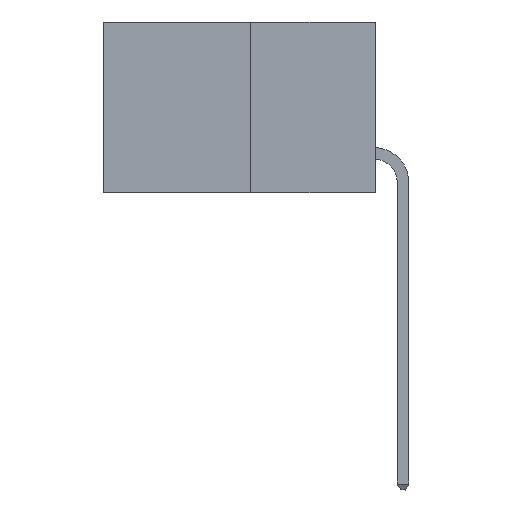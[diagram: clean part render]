
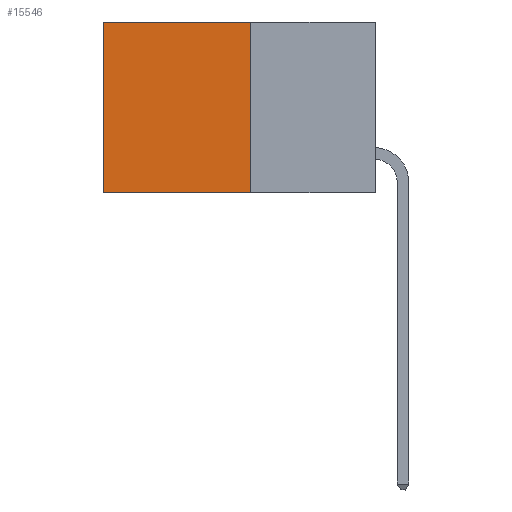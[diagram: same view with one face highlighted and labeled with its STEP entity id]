
A CAD part, left-side view. The second image highlights one B-rep face of the part: STEP entity #15546.
In plain terms, the highlighted planar face has unit normal (-1, 0, 0).
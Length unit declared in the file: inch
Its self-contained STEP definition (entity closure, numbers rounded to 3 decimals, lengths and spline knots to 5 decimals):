
#466 = DIRECTION ( 'NONE',  ( 0., 0., -1. ) ) ;
#811 = CARTESIAN_POINT ( 'NONE',  ( 0.277, 0.27, -0.37 ) ) ;
#1343 = VERTEX_POINT ( 'NONE', #15379 ) ;
#1377 = CARTESIAN_POINT ( 'NONE',  ( 0.277, 0.27, 0. ) ) ;
#2199 = DIRECTION ( 'NONE',  ( 0., 0., -1. ) ) ;
#2752 = EDGE_CURVE ( 'NONE', #14005, #12469, #15935, .T. ) ;
#4328 = VECTOR ( 'NONE', #6142, 39.37008 ) ;
#4479 = LINE ( 'NONE', #12150, #11175 ) ;
#4634 = EDGE_CURVE ( 'NONE', #8084, #1343, #10798, .T. ) ;
#4691 = CARTESIAN_POINT ( 'NONE',  ( 0.277, 0.27, -0.37 ) ) ;
#4989 = AXIS2_PLACEMENT_3D ( 'NONE', #811, #9878, #2199 ) ;
#5261 = ORIENTED_EDGE ( 'NONE', *, *, #2752, .F. ) ;
#5404 = EDGE_CURVE ( 'NONE', #8084, #14005, #16242, .T. ) ;
#5988 = ORIENTED_EDGE ( 'NONE', *, *, #4634, .T. ) ;
#6006 = ORIENTED_EDGE ( 'NONE', *, *, #5404, .F. ) ;
#6142 = DIRECTION ( 'NONE',  ( 0., 1., 0. ) ) ;
#7275 = ORIENTED_EDGE ( 'NONE', *, *, #8426, .T. ) ;
#8084 = VERTEX_POINT ( 'NONE', #1377 ) ;
#8426 = EDGE_CURVE ( 'NONE', #1343, #12469, #4479, .T. ) ;
#9634 = DIRECTION ( 'NONE',  ( 0., 0., -1. ) ) ;
#9728 = CARTESIAN_POINT ( 'NONE',  ( 0.277, 0.59, -0.37 ) ) ;
#9786 = VECTOR ( 'NONE', #9634, 39.37008 ) ;
#9875 = FACE_OUTER_BOUND ( 'NONE', #14881, .T. ) ;
#9878 = DIRECTION ( 'NONE',  ( 1., 0., 0. ) ) ;
#10403 = VECTOR ( 'NONE', #14454, 39.37008 ) ;
#10744 = CARTESIAN_POINT ( 'NONE',  ( 0.277, 0.27, -0.37 ) ) ;
#10798 = LINE ( 'NONE', #14337, #10403 ) ;
#11175 = VECTOR ( 'NONE', #466, 39.37008 ) ;
#12150 = CARTESIAN_POINT ( 'NONE',  ( 0.277, 0.59, -0.37 ) ) ;
#12469 = VERTEX_POINT ( 'NONE', #9728 ) ;
#13472 = CARTESIAN_POINT ( 'NONE',  ( 0.277, 0.27, -0.37 ) ) ;
#14005 = VERTEX_POINT ( 'NONE', #10744 ) ;
#14337 = CARTESIAN_POINT ( 'NONE',  ( 0.277, 0.27, 0. ) ) ;
#14454 = DIRECTION ( 'NONE',  ( 0., 1., 0. ) ) ;
#14881 = EDGE_LOOP ( 'NONE', ( #7275, #5261, #6006, #5988 ) ) ;
#15379 = CARTESIAN_POINT ( 'NONE',  ( 0.277, 0.59, 0. ) ) ;
#15546 = ADVANCED_FACE ( 'NONE', ( #9875 ), #15929, .F. ) ;
#15929 = PLANE ( 'NONE',  #4989 ) ;
#15935 = LINE ( 'NONE', #13472, #4328 ) ;
#16242 = LINE ( 'NONE', #4691, #9786 ) ;
